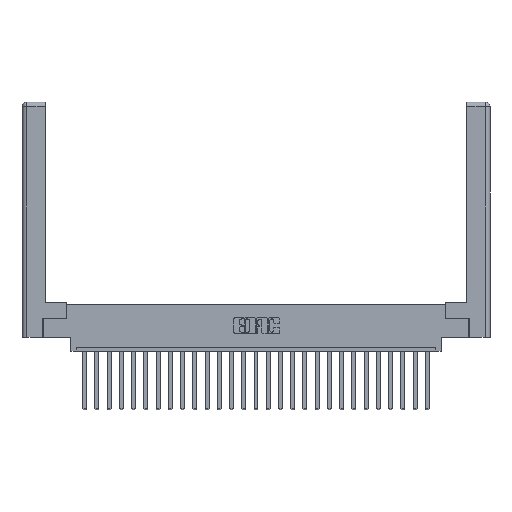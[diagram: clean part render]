
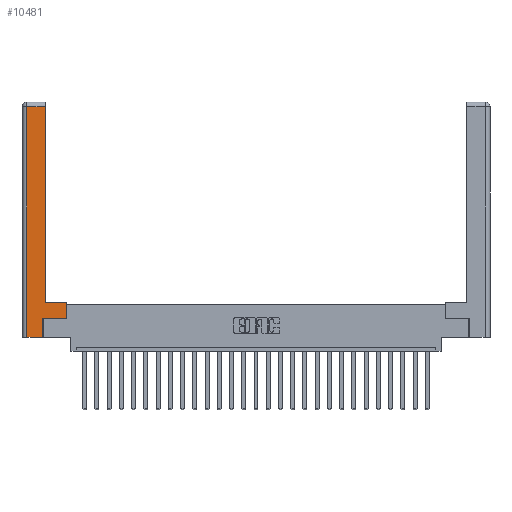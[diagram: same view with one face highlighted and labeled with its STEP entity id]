
A CAD part, top view. The second image highlights one B-rep face of the part: STEP entity #10481.
In plain terms, the highlighted planar face has unit normal (0, 0, 1).
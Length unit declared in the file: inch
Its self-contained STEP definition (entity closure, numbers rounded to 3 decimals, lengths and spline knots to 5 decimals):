
#462 = EDGE_CURVE ( 'NONE', #5570, #11050, #25613, .T. ) ;
#977 = LINE ( 'NONE', #23574, #3144 ) ;
#1515 = VERTEX_POINT ( 'NONE', #25374 ) ;
#1743 = CARTESIAN_POINT ( 'NONE',  ( 0., 0., 0. ) ) ;
#1854 = EDGE_LOOP ( 'NONE', ( #10715, #9615, #19277, #19597, #1929, #3578, #25191, #15976 ) ) ;
#1929 = ORIENTED_EDGE ( 'NONE', *, *, #11952, .T. ) ;
#2121 = LINE ( 'NONE', #25791, #9603 ) ;
#2650 = AXIS2_PLACEMENT_3D ( 'NONE', #1743, #3645, #11857 ) ;
#2663 = CARTESIAN_POINT ( 'NONE',  ( 0.565, 0.245, 0. ) ) ;
#3128 = DIRECTION ( 'NONE',  ( 0., 1., 0. ) ) ;
#3144 = VECTOR ( 'NONE', #5806, 39.37008 ) ;
#3578 = ORIENTED_EDGE ( 'NONE', *, *, #14555, .T. ) ;
#3597 = CARTESIAN_POINT ( 'NONE',  ( 0.565, 0.45, 0. ) ) ;
#3645 = DIRECTION ( 'NONE',  ( 0., 0., -1. ) ) ;
#4162 = DIRECTION ( 'NONE',  ( 1., 0., 0. ) ) ;
#4578 = VECTOR ( 'NONE', #8101, 39.37008 ) ;
#4804 = LINE ( 'NONE', #2663, #19156 ) ;
#5045 = EDGE_CURVE ( 'NONE', #10696, #7440, #977, .T. ) ;
#5396 = CARTESIAN_POINT ( 'NONE',  ( 0.295, 3., 0. ) ) ;
#5570 = VERTEX_POINT ( 'NONE', #25714 ) ;
#5806 = DIRECTION ( 'NONE',  ( -1., 0., 0. ) ) ;
#5935 = LINE ( 'NONE', #25690, #6855 ) ;
#6565 = EDGE_CURVE ( 'NONE', #8146, #5570, #2121, .T. ) ;
#6612 = LINE ( 'NONE', #3597, #15052 ) ;
#6752 = LINE ( 'NONE', #5396, #25156 ) ;
#6855 = VECTOR ( 'NONE', #15849, 39.37008 ) ;
#7440 = VERTEX_POINT ( 'NONE', #14864 ) ;
#8006 = DIRECTION ( 'NONE',  ( 0., -1., 0. ) ) ;
#8101 = DIRECTION ( 'NONE',  ( -1., 0., 0. ) ) ;
#8146 = VERTEX_POINT ( 'NONE', #23778 ) ;
#8538 = CARTESIAN_POINT ( 'NONE',  ( 0.565, 0.45, 0. ) ) ;
#9603 = VECTOR ( 'NONE', #8006, 39.37008 ) ;
#9615 = ORIENTED_EDGE ( 'NONE', *, *, #25219, .T. ) ;
#9899 = LINE ( 'NONE', #14133, #4578 ) ;
#9970 = CARTESIAN_POINT ( 'NONE',  ( 0.565, 0.245, 0. ) ) ;
#10481 = ADVANCED_FACE ( 'NONE', ( #22805 ), #21965, .F. ) ;
#10696 = VERTEX_POINT ( 'NONE', #8538 ) ;
#10715 = ORIENTED_EDGE ( 'NONE', *, *, #25239, .T. ) ;
#11050 = VERTEX_POINT ( 'NONE', #17599 ) ;
#11377 = CARTESIAN_POINT ( 'NONE',  ( 0.265, 0.245, 0. ) ) ;
#11857 = DIRECTION ( 'NONE',  ( -1., 0., 0. ) ) ;
#11952 = EDGE_CURVE ( 'NONE', #11050, #22731, #5935, .T. ) ;
#14133 = CARTESIAN_POINT ( 'NONE',  ( 0.0615, 2.94, 0. ) ) ;
#14555 = EDGE_CURVE ( 'NONE', #22731, #17760, #4804, .T. ) ;
#14864 = CARTESIAN_POINT ( 'NONE',  ( 0.295, 0.45, 0. ) ) ;
#15052 = VECTOR ( 'NONE', #23549, 39.37008 ) ;
#15849 = DIRECTION ( 'NONE',  ( 0., 1., 0. ) ) ;
#15976 = ORIENTED_EDGE ( 'NONE', *, *, #5045, .T. ) ;
#16035 = CARTESIAN_POINT ( 'NONE',  ( 0.265, 0., 0. ) ) ;
#16589 = EDGE_CURVE ( 'NONE', #17760, #10696, #6612, .T. ) ;
#17599 = CARTESIAN_POINT ( 'NONE',  ( 0.265, 0., 0. ) ) ;
#17760 = VERTEX_POINT ( 'NONE', #9970 ) ;
#18430 = VECTOR ( 'NONE', #4162, 39.37008 ) ;
#18787 = DIRECTION ( 'NONE',  ( 1., 0., 0. ) ) ;
#19156 = VECTOR ( 'NONE', #18787, 39.37008 ) ;
#19277 = ORIENTED_EDGE ( 'NONE', *, *, #6565, .T. ) ;
#19597 = ORIENTED_EDGE ( 'NONE', *, *, #462, .T. ) ;
#21965 = PLANE ( 'NONE',  #2650 ) ;
#22731 = VERTEX_POINT ( 'NONE', #11377 ) ;
#22805 = FACE_OUTER_BOUND ( 'NONE', #1854, .T. ) ;
#23549 = DIRECTION ( 'NONE',  ( 0., 1., 0. ) ) ;
#23574 = CARTESIAN_POINT ( 'NONE',  ( 0.295, 0.45, 0. ) ) ;
#23778 = CARTESIAN_POINT ( 'NONE',  ( 0.0615, 2.94, 0. ) ) ;
#25156 = VECTOR ( 'NONE', #3128, 39.37008 ) ;
#25191 = ORIENTED_EDGE ( 'NONE', *, *, #16589, .T. ) ;
#25219 = EDGE_CURVE ( 'NONE', #1515, #8146, #9899, .T. ) ;
#25239 = EDGE_CURVE ( 'NONE', #7440, #1515, #6752, .T. ) ;
#25374 = CARTESIAN_POINT ( 'NONE',  ( 0.295, 2.94, 0. ) ) ;
#25613 = LINE ( 'NONE', #16035, #18430 ) ;
#25690 = CARTESIAN_POINT ( 'NONE',  ( 0.265, 0.245, 0. ) ) ;
#25714 = CARTESIAN_POINT ( 'NONE',  ( 0.0615, 0., 0. ) ) ;
#25791 = CARTESIAN_POINT ( 'NONE',  ( 0.0615, 0., 0. ) ) ;
